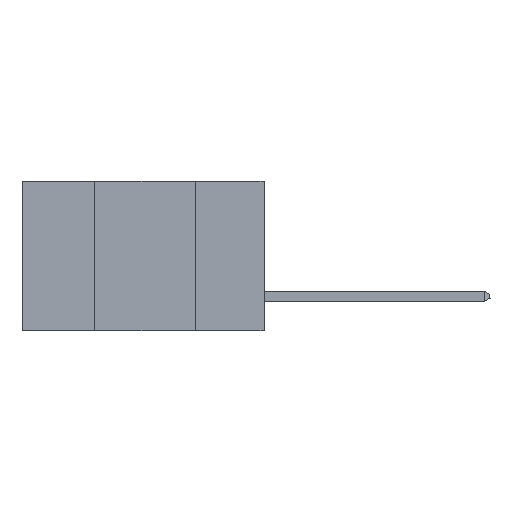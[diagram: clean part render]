
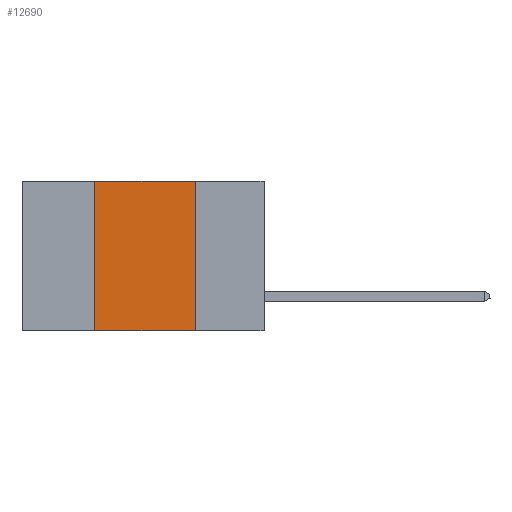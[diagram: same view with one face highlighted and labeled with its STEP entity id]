
A CAD part, left-side view. The second image highlights one B-rep face of the part: STEP entity #12690.
In plain terms, the highlighted planar face has unit normal (-1, 0, 0).
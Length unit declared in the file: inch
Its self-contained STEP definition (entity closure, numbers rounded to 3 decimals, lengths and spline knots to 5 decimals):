
#789 = ORIENTED_EDGE ( 'NONE', *, *, #12358, .F. ) ;
#929 = CARTESIAN_POINT ( 'NONE',  ( 0., 0.6, -0.37 ) ) ;
#1008 = LINE ( 'NONE', #6258, #14840 ) ;
#1024 = DIRECTION ( 'NONE',  ( 1., 0., 0. ) ) ;
#1509 = CARTESIAN_POINT ( 'NONE',  ( 0., 0.17, -0.37 ) ) ;
#1725 = DIRECTION ( 'NONE',  ( 0., 0., 1. ) ) ;
#1790 = ORIENTED_EDGE ( 'NONE', *, *, #12224, .F. ) ;
#1999 = VERTEX_POINT ( 'NONE', #7380 ) ;
#2003 = VERTEX_POINT ( 'NONE', #1509 ) ;
#2055 = LINE ( 'NONE', #929, #12918 ) ;
#2597 = DIRECTION ( 'NONE',  ( 0., -1., 0. ) ) ;
#2881 = EDGE_LOOP ( 'NONE', ( #10434, #1790, #789, #14575 ) ) ;
#3611 = EDGE_CURVE ( 'NONE', #1999, #2003, #2055, .T. ) ;
#4096 = EDGE_CURVE ( 'NONE', #13903, #2003, #6521, .T. ) ;
#6258 = CARTESIAN_POINT ( 'NONE',  ( 0., 0.6, 0. ) ) ;
#6521 = LINE ( 'NONE', #12611, #14768 ) ;
#6989 = CARTESIAN_POINT ( 'NONE',  ( 0., 0.17, 0. ) ) ;
#7177 = VECTOR ( 'NONE', #1725, 39.37008 ) ;
#7380 = CARTESIAN_POINT ( 'NONE',  ( 0., 0.42, -0.37 ) ) ;
#7553 = LINE ( 'NONE', #11189, #7177 ) ;
#7711 = VERTEX_POINT ( 'NONE', #13707 ) ;
#8878 = FACE_OUTER_BOUND ( 'NONE', #2881, .T. ) ;
#9205 = DIRECTION ( 'NONE',  ( 0., 0., -1. ) ) ;
#9253 = AXIS2_PLACEMENT_3D ( 'NONE', #14027, #1024, #9409 ) ;
#9409 = DIRECTION ( 'NONE',  ( 0., 0., -1. ) ) ;
#9507 = PLANE ( 'NONE',  #9253 ) ;
#10434 = ORIENTED_EDGE ( 'NONE', *, *, #4096, .F. ) ;
#11189 = CARTESIAN_POINT ( 'NONE',  ( 0., 0.42, -0.37 ) ) ;
#11748 = DIRECTION ( 'NONE',  ( 0., -1., 0. ) ) ;
#12224 = EDGE_CURVE ( 'NONE', #7711, #13903, #1008, .T. ) ;
#12358 = EDGE_CURVE ( 'NONE', #1999, #7711, #7553, .T. ) ;
#12611 = CARTESIAN_POINT ( 'NONE',  ( 0., 0.17, -0.37 ) ) ;
#12690 = ADVANCED_FACE ( 'NONE', ( #8878 ), #9507, .F. ) ;
#12918 = VECTOR ( 'NONE', #11748, 39.37008 ) ;
#13707 = CARTESIAN_POINT ( 'NONE',  ( 0., 0.42, 0. ) ) ;
#13903 = VERTEX_POINT ( 'NONE', #6989 ) ;
#14027 = CARTESIAN_POINT ( 'NONE',  ( 0., 0.6, 0. ) ) ;
#14575 = ORIENTED_EDGE ( 'NONE', *, *, #3611, .T. ) ;
#14768 = VECTOR ( 'NONE', #9205, 39.37008 ) ;
#14840 = VECTOR ( 'NONE', #2597, 39.37008 ) ;
